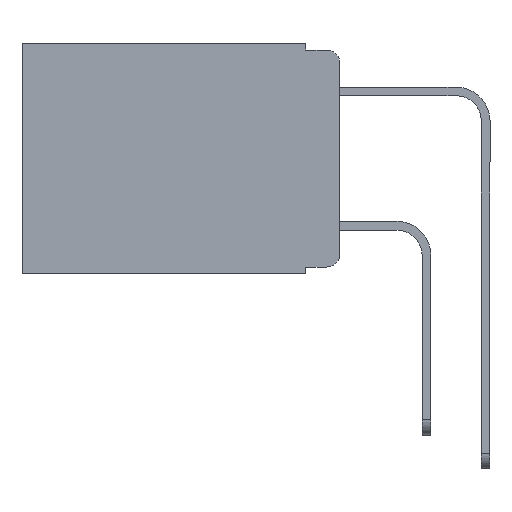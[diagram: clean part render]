
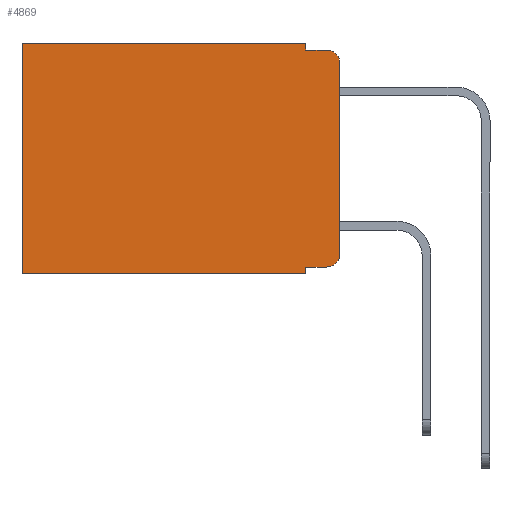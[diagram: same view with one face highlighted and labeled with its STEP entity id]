
A CAD part, left-side view. The second image highlights one B-rep face of the part: STEP entity #4869.
In plain terms, the highlighted planar face has unit normal (-1, 0, 0).
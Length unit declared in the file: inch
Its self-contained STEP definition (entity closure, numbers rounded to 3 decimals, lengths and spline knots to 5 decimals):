
#37 = DIRECTION ( 'NONE',  ( 0., 0., -1. ) ) ;
#114 = AXIS2_PLACEMENT_3D ( 'NONE', #11240, #4859, #4847 ) ;
#414 = VERTEX_POINT ( 'NONE', #8076 ) ;
#429 = VERTEX_POINT ( 'NONE', #1897 ) ;
#703 = VECTOR ( 'NONE', #5503, 39.37008 ) ;
#749 = ORIENTED_EDGE ( 'NONE', *, *, #10518, .F. ) ;
#985 = LINE ( 'NONE', #7032, #3439 ) ;
#1070 = DIRECTION ( 'NONE',  ( 0., 0., -1. ) ) ;
#1415 = ORIENTED_EDGE ( 'NONE', *, *, #12792, .T. ) ;
#1510 = LINE ( 'NONE', #4834, #5889 ) ;
#1897 = CARTESIAN_POINT ( 'NONE',  ( 0.298, 0.051, -0.333 ) ) ;
#2437 = CARTESIAN_POINT ( 'NONE',  ( 0.298, 0., -0.03 ) ) ;
#2633 = VERTEX_POINT ( 'NONE', #2437 ) ;
#2951 = CARTESIAN_POINT ( 'NONE',  ( 0.298, 0.051, -0.333 ) ) ;
#3030 = CARTESIAN_POINT ( 'NONE',  ( 0.298, 0.051, 0. ) ) ;
#3439 = VECTOR ( 'NONE', #4148, 39.37008 ) ;
#3527 = ORIENTED_EDGE ( 'NONE', *, *, #8180, .T. ) ;
#3615 = FACE_OUTER_BOUND ( 'NONE', #10354, .T. ) ;
#3851 = ORIENTED_EDGE ( 'NONE', *, *, #10610, .F. ) ;
#3878 = AXIS2_PLACEMENT_3D ( 'NONE', #5597, #12344, #6590 ) ;
#4005 = AXIS2_PLACEMENT_3D ( 'NONE', #12799, #7057, #1070 ) ;
#4116 = VERTEX_POINT ( 'NONE', #9159 ) ;
#4119 = VERTEX_POINT ( 'NONE', #5607 ) ;
#4148 = DIRECTION ( 'NONE',  ( 0., 1., 0. ) ) ;
#4225 = CARTESIAN_POINT ( 'NONE',  ( 0.298, 0.02, -0.333 ) ) ;
#4243 = DIRECTION ( 'NONE',  ( 0., -1., 0. ) ) ;
#4252 = VECTOR ( 'NONE', #5954, 39.37008 ) ;
#4265 = DIRECTION ( 'NONE',  ( 0., 0., -1. ) ) ;
#4291 = CARTESIAN_POINT ( 'NONE',  ( 0.298, 0.02, -0.01 ) ) ;
#4328 = ORIENTED_EDGE ( 'NONE', *, *, #11680, .T. ) ;
#4367 = VECTOR ( 'NONE', #5931, 39.37008 ) ;
#4403 = ORIENTED_EDGE ( 'NONE', *, *, #9094, .T. ) ;
#4425 = LINE ( 'NONE', #11961, #9024 ) ;
#4535 = CARTESIAN_POINT ( 'NONE',  ( 0.298, 0.473, 0. ) ) ;
#4666 = LINE ( 'NONE', #3030, #4367 ) ;
#4702 = ORIENTED_EDGE ( 'NONE', *, *, #11888, .F. ) ;
#4834 = CARTESIAN_POINT ( 'NONE',  ( 0.298, 0., 0. ) ) ;
#4847 = DIRECTION ( 'NONE',  ( 0., 0., -1. ) ) ;
#4859 = DIRECTION ( 'NONE',  ( 1., 0., 0. ) ) ;
#4865 = VERTEX_POINT ( 'NONE', #4291 ) ;
#4869 = ADVANCED_FACE ( 'NONE', ( #3615 ), #11301, .F. ) ;
#4873 = EDGE_CURVE ( 'NONE', #2633, #4119, #1510, .T. ) ;
#4887 = VERTEX_POINT ( 'NONE', #4225 ) ;
#5390 = VECTOR ( 'NONE', #4243, 39.37008 ) ;
#5477 = CARTESIAN_POINT ( 'NONE',  ( 0.298, 0.051, -0.01 ) ) ;
#5503 = DIRECTION ( 'NONE',  ( 0., 0., -1. ) ) ;
#5536 = LINE ( 'NONE', #2951, #5842 ) ;
#5597 = CARTESIAN_POINT ( 'NONE',  ( 0.298, 0.02, -0.313 ) ) ;
#5607 = CARTESIAN_POINT ( 'NONE',  ( 0.298, 0., -0.313 ) ) ;
#5678 = LINE ( 'NONE', #11983, #5390 ) ;
#5842 = VECTOR ( 'NONE', #8838, 39.37008 ) ;
#5889 = VECTOR ( 'NONE', #4265, 39.37008 ) ;
#5931 = DIRECTION ( 'NONE',  ( 0., 0., -1. ) ) ;
#5954 = DIRECTION ( 'NONE',  ( 0., 1., 0. ) ) ;
#6590 = DIRECTION ( 'NONE',  ( 0., 0., -1. ) ) ;
#7032 = CARTESIAN_POINT ( 'NONE',  ( 0.298, 0., -0.343 ) ) ;
#7057 = DIRECTION ( 'NONE',  ( -1., 0., 0. ) ) ;
#7453 = ORIENTED_EDGE ( 'NONE', *, *, #4873, .F. ) ;
#7521 = VERTEX_POINT ( 'NONE', #5477 ) ;
#8076 = CARTESIAN_POINT ( 'NONE',  ( 0.298, 0.051, -0.343 ) ) ;
#8180 = EDGE_CURVE ( 'NONE', #8870, #4116, #11269, .T. ) ;
#8579 = EDGE_CURVE ( 'NONE', #11654, #7521, #4425, .T. ) ;
#8838 = DIRECTION ( 'NONE',  ( 0., -1., 0. ) ) ;
#8870 = VERTEX_POINT ( 'NONE', #10528 ) ;
#9024 = VECTOR ( 'NONE', #37, 39.37008 ) ;
#9094 = EDGE_CURVE ( 'NONE', #11654, #8870, #9469, .T. ) ;
#9159 = CARTESIAN_POINT ( 'NONE',  ( 0.298, 0.473, -0.343 ) ) ;
#9460 = CIRCLE ( 'NONE', #4005, 0.02 ) ;
#9469 = LINE ( 'NONE', #11745, #4252 ) ;
#9483 = EDGE_CURVE ( 'NONE', #2633, #4865, #9460, .T. ) ;
#10154 = ORIENTED_EDGE ( 'NONE', *, *, #8579, .F. ) ;
#10354 = EDGE_LOOP ( 'NONE', ( #7453, #12284, #4702, #10154, #4403, #3527, #3851, #749, #4328, #1415 ) ) ;
#10518 = EDGE_CURVE ( 'NONE', #429, #414, #4666, .T. ) ;
#10528 = CARTESIAN_POINT ( 'NONE',  ( 0.298, 0.473, 0. ) ) ;
#10610 = EDGE_CURVE ( 'NONE', #414, #4116, #985, .T. ) ;
#11240 = CARTESIAN_POINT ( 'NONE',  ( 0.298, 0., 0. ) ) ;
#11269 = LINE ( 'NONE', #4535, #703 ) ;
#11301 = PLANE ( 'NONE',  #114 ) ;
#11654 = VERTEX_POINT ( 'NONE', #12543 ) ;
#11680 = EDGE_CURVE ( 'NONE', #429, #4887, #5536, .T. ) ;
#11745 = CARTESIAN_POINT ( 'NONE',  ( 0.298, 0., 0. ) ) ;
#11862 = CIRCLE ( 'NONE', #3878, 0.02 ) ;
#11888 = EDGE_CURVE ( 'NONE', #7521, #4865, #5678, .T. ) ;
#11961 = CARTESIAN_POINT ( 'NONE',  ( 0.298, 0.051, 0. ) ) ;
#11983 = CARTESIAN_POINT ( 'NONE',  ( 0.298, 0.051, -0.01 ) ) ;
#12284 = ORIENTED_EDGE ( 'NONE', *, *, #9483, .T. ) ;
#12344 = DIRECTION ( 'NONE',  ( -1., 0., 0. ) ) ;
#12543 = CARTESIAN_POINT ( 'NONE',  ( 0.298, 0.051, 0. ) ) ;
#12792 = EDGE_CURVE ( 'NONE', #4887, #4119, #11862, .T. ) ;
#12799 = CARTESIAN_POINT ( 'NONE',  ( 0.298, 0.02, -0.03 ) ) ;
